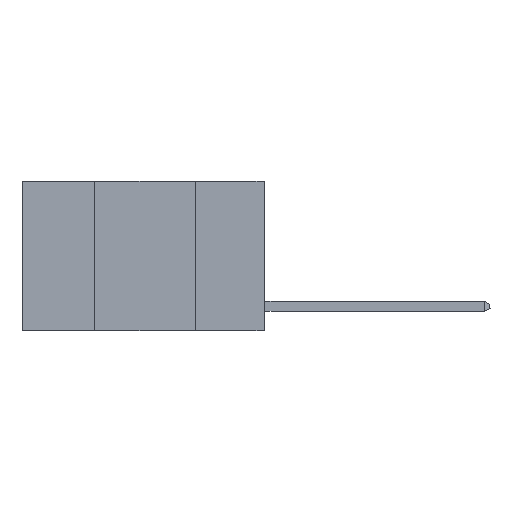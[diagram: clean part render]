
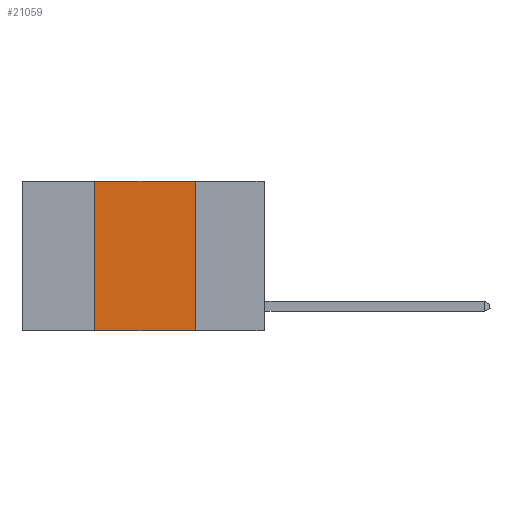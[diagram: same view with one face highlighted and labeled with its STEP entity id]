
A CAD part, left-side view. The second image highlights one B-rep face of the part: STEP entity #21059.
In plain terms, the highlighted planar face has unit normal (-1, 0, 0).
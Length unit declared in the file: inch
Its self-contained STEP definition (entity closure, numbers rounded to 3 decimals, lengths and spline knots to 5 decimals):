
#155 = EDGE_CURVE ( 'NONE', #6346, #4635, #8171, .T. ) ;
#213 = DIRECTION ( 'NONE',  ( 0., -1., 0. ) ) ;
#1191 = DIRECTION ( 'NONE',  ( 1., 0., 0. ) ) ;
#1688 = LINE ( 'NONE', #17906, #13979 ) ;
#2048 = CARTESIAN_POINT ( 'NONE',  ( 0., 0.17, -0.37 ) ) ;
#2359 = PLANE ( 'NONE',  #17772 ) ;
#3045 = ORIENTED_EDGE ( 'NONE', *, *, #12216, .T. ) ;
#3678 = LINE ( 'NONE', #10215, #14122 ) ;
#4039 = VECTOR ( 'NONE', #15332, 39.37008 ) ;
#4635 = VERTEX_POINT ( 'NONE', #21030 ) ;
#6115 = ORIENTED_EDGE ( 'NONE', *, *, #14687, .F. ) ;
#6118 = VECTOR ( 'NONE', #8489, 39.37008 ) ;
#6346 = VERTEX_POINT ( 'NONE', #20134 ) ;
#7460 = VERTEX_POINT ( 'NONE', #14721 ) ;
#8171 = LINE ( 'NONE', #14679, #6118 ) ;
#8489 = DIRECTION ( 'NONE',  ( 0., -1., 0. ) ) ;
#9531 = EDGE_CURVE ( 'NONE', #4635, #10056, #15112, .T. ) ;
#10056 = VERTEX_POINT ( 'NONE', #2048 ) ;
#10215 = CARTESIAN_POINT ( 'NONE',  ( 0., 0.42, 0. ) ) ;
#10313 = CARTESIAN_POINT ( 'NONE',  ( 0., 0.17, 0. ) ) ;
#12216 = EDGE_CURVE ( 'NONE', #7460, #10056, #1688, .T. ) ;
#13590 = ORIENTED_EDGE ( 'NONE', *, *, #155, .F. ) ;
#13900 = DIRECTION ( 'NONE',  ( 0., 0., -1. ) ) ;
#13979 = VECTOR ( 'NONE', #213, 39.37008 ) ;
#14122 = VECTOR ( 'NONE', #16855, 39.37008 ) ;
#14679 = CARTESIAN_POINT ( 'NONE',  ( 0., 0.6, 0. ) ) ;
#14687 = EDGE_CURVE ( 'NONE', #7460, #6346, #3678, .T. ) ;
#14721 = CARTESIAN_POINT ( 'NONE',  ( 0., 0.42, -0.37 ) ) ;
#15112 = LINE ( 'NONE', #10313, #4039 ) ;
#15332 = DIRECTION ( 'NONE',  ( 0., 0., -1. ) ) ;
#15532 = CARTESIAN_POINT ( 'NONE',  ( 0., 0.6, 0. ) ) ;
#15842 = EDGE_LOOP ( 'NONE', ( #19920, #13590, #6115, #3045 ) ) ;
#16855 = DIRECTION ( 'NONE',  ( 0., 0., 1. ) ) ;
#17772 = AXIS2_PLACEMENT_3D ( 'NONE', #15532, #1191, #13900 ) ;
#17906 = CARTESIAN_POINT ( 'NONE',  ( 0., 0.6, -0.37 ) ) ;
#19008 = FACE_OUTER_BOUND ( 'NONE', #15842, .T. ) ;
#19920 = ORIENTED_EDGE ( 'NONE', *, *, #9531, .F. ) ;
#20134 = CARTESIAN_POINT ( 'NONE',  ( 0., 0.42, 0. ) ) ;
#21030 = CARTESIAN_POINT ( 'NONE',  ( 0., 0.17, 0. ) ) ;
#21059 = ADVANCED_FACE ( 'NONE', ( #19008 ), #2359, .F. ) ;
